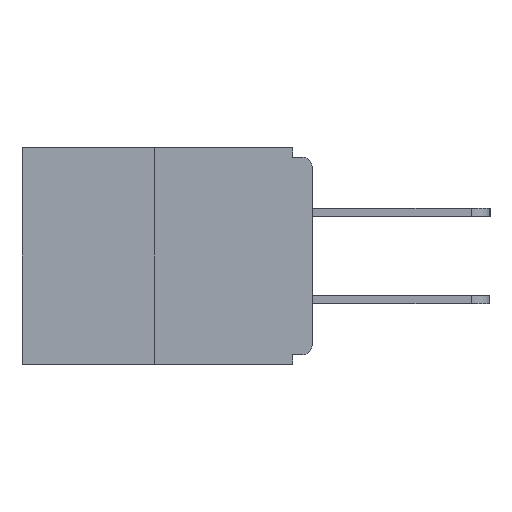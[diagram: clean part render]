
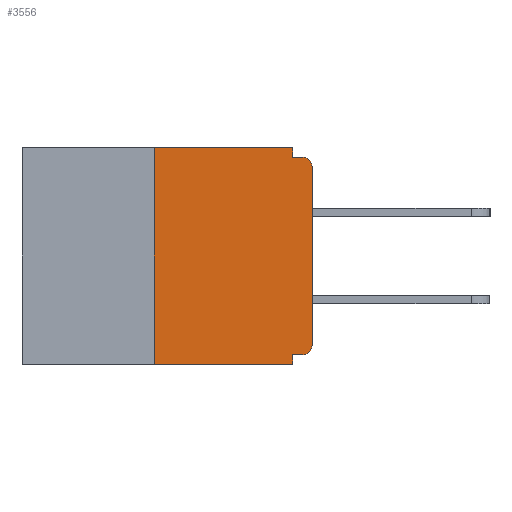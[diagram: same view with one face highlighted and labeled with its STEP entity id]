
A CAD part, left-side view. The second image highlights one B-rep face of the part: STEP entity #3556.
In plain terms, the highlighted planar face has unit normal (-1, 0, 0).
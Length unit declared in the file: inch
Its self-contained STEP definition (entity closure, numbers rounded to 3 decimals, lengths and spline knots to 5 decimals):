
#49 = DIRECTION ( 'NONE',  ( 0., 0., -1. ) ) ;
#68 = VERTEX_POINT ( 'NONE', #10982 ) ;
#224 = CARTESIAN_POINT ( 'NONE',  ( 0., 0., 0. ) ) ;
#542 = VECTOR ( 'NONE', #2564, 39.37008 ) ;
#733 = CARTESIAN_POINT ( 'NONE',  ( 0., 0.031, -0.343 ) ) ;
#1257 = DIRECTION ( 'NONE',  ( 0., -1., 0. ) ) ;
#1267 = ORIENTED_EDGE ( 'NONE', *, *, #8754, .F. ) ;
#1421 = LINE ( 'NONE', #224, #12818 ) ;
#1596 = CARTESIAN_POINT ( 'NONE',  ( 0., 0., -0.015 ) ) ;
#1784 = ORIENTED_EDGE ( 'NONE', *, *, #4947, .T. ) ;
#1811 = VECTOR ( 'NONE', #4316, 39.37008 ) ;
#1984 = DIRECTION ( 'NONE',  ( -1., 0., 0. ) ) ;
#2341 = VERTEX_POINT ( 'NONE', #13601 ) ;
#2345 = EDGE_CURVE ( 'NONE', #68, #9707, #10234, .T. ) ;
#2564 = DIRECTION ( 'NONE',  ( 0., -1., 0. ) ) ;
#2582 = VERTEX_POINT ( 'NONE', #10109 ) ;
#2590 = ORIENTED_EDGE ( 'NONE', *, *, #7462, .T. ) ;
#2616 = DIRECTION ( 'NONE',  ( 0., 0., -1. ) ) ;
#2694 = CARTESIAN_POINT ( 'NONE',  ( 0., 0.031, -0.343 ) ) ;
#3273 = AXIS2_PLACEMENT_3D ( 'NONE', #9838, #14916, #49 ) ;
#3556 = ADVANCED_FACE ( 'NONE', ( #6320 ), #10071, .F. ) ;
#3702 = AXIS2_PLACEMENT_3D ( 'NONE', #15488, #1984, #15724 ) ;
#3711 = CIRCLE ( 'NONE', #3702, 0.015 ) ;
#3722 = CARTESIAN_POINT ( 'NONE',  ( 0., 0.46, 0. ) ) ;
#3854 = CARTESIAN_POINT ( 'NONE',  ( 0., 0.46, 0. ) ) ;
#4143 = VERTEX_POINT ( 'NONE', #13517 ) ;
#4304 = CARTESIAN_POINT ( 'NONE',  ( 0., 0.015, -0.015 ) ) ;
#4316 = DIRECTION ( 'NONE',  ( 0., 0., -1. ) ) ;
#4463 = CARTESIAN_POINT ( 'NONE',  ( 0., 0.25, 0. ) ) ;
#4498 = ORIENTED_EDGE ( 'NONE', *, *, #13179, .F. ) ;
#4947 = EDGE_CURVE ( 'NONE', #2582, #5906, #13479, .T. ) ;
#5340 = DIRECTION ( 'NONE',  ( 0., 0., -1. ) ) ;
#5449 = CARTESIAN_POINT ( 'NONE',  ( 0., 0., -0.313 ) ) ;
#5906 = VERTEX_POINT ( 'NONE', #4304 ) ;
#6002 = LINE ( 'NONE', #9598, #11822 ) ;
#6009 = EDGE_CURVE ( 'NONE', #6759, #15787, #9466, .T. ) ;
#6027 = VECTOR ( 'NONE', #11997, 39.37008 ) ;
#6103 = ORIENTED_EDGE ( 'NONE', *, *, #13457, .F. ) ;
#6320 = FACE_OUTER_BOUND ( 'NONE', #12432, .T. ) ;
#6358 = VERTEX_POINT ( 'NONE', #5449 ) ;
#6481 = CARTESIAN_POINT ( 'NONE',  ( 0., 0.031, 0. ) ) ;
#6759 = VERTEX_POINT ( 'NONE', #12780 ) ;
#6764 = ORIENTED_EDGE ( 'NONE', *, *, #6009, .T. ) ;
#6928 = LINE ( 'NONE', #4463, #6027 ) ;
#7089 = VERTEX_POINT ( 'NONE', #10035 ) ;
#7462 = EDGE_CURVE ( 'NONE', #6358, #2582, #1421, .T. ) ;
#8575 = EDGE_CURVE ( 'NONE', #4143, #6358, #3711, .T. ) ;
#8754 = EDGE_CURVE ( 'NONE', #4143, #2341, #6002, .T. ) ;
#8791 = DIRECTION ( 'NONE',  ( 0., 0., 1. ) ) ;
#9466 = LINE ( 'NONE', #12003, #13352 ) ;
#9598 = CARTESIAN_POINT ( 'NONE',  ( 0., 0., -0.328 ) ) ;
#9613 = DIRECTION ( 'NONE',  ( 0., -1., 0. ) ) ;
#9707 = VERTEX_POINT ( 'NONE', #12346 ) ;
#9838 = CARTESIAN_POINT ( 'NONE',  ( 0., 0.015, -0.03 ) ) ;
#9934 = LINE ( 'NONE', #3722, #15429 ) ;
#10035 = CARTESIAN_POINT ( 'NONE',  ( 0., 0.25, 0. ) ) ;
#10071 = PLANE ( 'NONE',  #12273 ) ;
#10109 = CARTESIAN_POINT ( 'NONE',  ( 0., 0., -0.03 ) ) ;
#10234 = LINE ( 'NONE', #6481, #11694 ) ;
#10271 = LINE ( 'NONE', #1596, #542 ) ;
#10321 = ORIENTED_EDGE ( 'NONE', *, *, #15440, .F. ) ;
#10675 = ORIENTED_EDGE ( 'NONE', *, *, #8575, .T. ) ;
#10909 = DIRECTION ( 'NONE',  ( 0., 1., 0. ) ) ;
#10982 = CARTESIAN_POINT ( 'NONE',  ( 0., 0.031, 0. ) ) ;
#11694 = VECTOR ( 'NONE', #5340, 39.37008 ) ;
#11822 = VECTOR ( 'NONE', #10909, 39.37008 ) ;
#11997 = DIRECTION ( 'NONE',  ( 0., 0., 1. ) ) ;
#12003 = CARTESIAN_POINT ( 'NONE',  ( 0., 0.46, -0.343 ) ) ;
#12273 = AXIS2_PLACEMENT_3D ( 'NONE', #3854, #13834, #2616 ) ;
#12346 = CARTESIAN_POINT ( 'NONE',  ( 0., 0.031, -0.015 ) ) ;
#12432 = EDGE_LOOP ( 'NONE', ( #10321, #14877, #6764, #4498, #1267, #10675, #2590, #1784, #6103, #14350 ) ) ;
#12780 = CARTESIAN_POINT ( 'NONE',  ( 0., 0.25, -0.343 ) ) ;
#12818 = VECTOR ( 'NONE', #8791, 39.37008 ) ;
#13179 = EDGE_CURVE ( 'NONE', #2341, #15787, #14450, .T. ) ;
#13352 = VECTOR ( 'NONE', #9613, 39.37008 ) ;
#13457 = EDGE_CURVE ( 'NONE', #9707, #5906, #10271, .T. ) ;
#13479 = CIRCLE ( 'NONE', #3273, 0.015 ) ;
#13517 = CARTESIAN_POINT ( 'NONE',  ( 0., 0.015, -0.328 ) ) ;
#13601 = CARTESIAN_POINT ( 'NONE',  ( 0., 0.031, -0.328 ) ) ;
#13607 = EDGE_CURVE ( 'NONE', #6759, #7089, #6928, .T. ) ;
#13834 = DIRECTION ( 'NONE',  ( 1., 0., 0. ) ) ;
#14350 = ORIENTED_EDGE ( 'NONE', *, *, #2345, .F. ) ;
#14450 = LINE ( 'NONE', #733, #1811 ) ;
#14877 = ORIENTED_EDGE ( 'NONE', *, *, #13607, .F. ) ;
#14916 = DIRECTION ( 'NONE',  ( -1., 0., 0. ) ) ;
#15429 = VECTOR ( 'NONE', #1257, 39.37008 ) ;
#15440 = EDGE_CURVE ( 'NONE', #7089, #68, #9934, .T. ) ;
#15488 = CARTESIAN_POINT ( 'NONE',  ( 0., 0.015, -0.313 ) ) ;
#15724 = DIRECTION ( 'NONE',  ( 0., 0., -1. ) ) ;
#15787 = VERTEX_POINT ( 'NONE', #2694 ) ;
